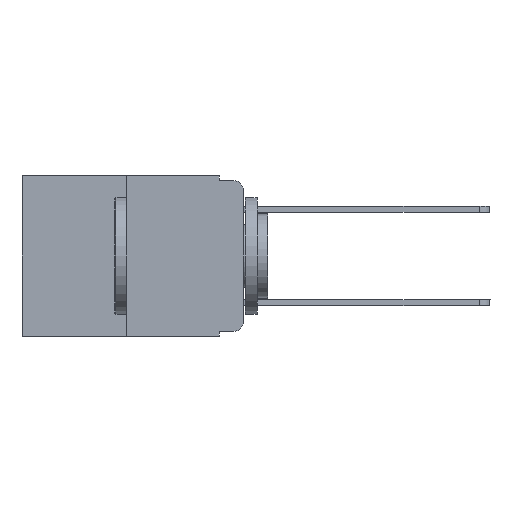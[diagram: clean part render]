
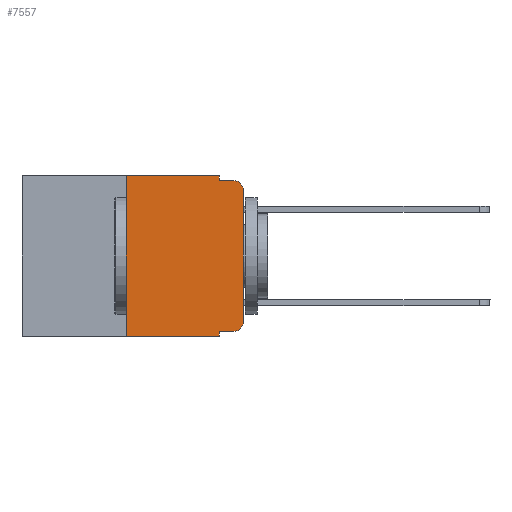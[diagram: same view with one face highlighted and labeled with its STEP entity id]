
A CAD part, left-side view. The second image highlights one B-rep face of the part: STEP entity #7557.
In plain terms, the highlighted planar face has unit normal (-1, 0, 0).
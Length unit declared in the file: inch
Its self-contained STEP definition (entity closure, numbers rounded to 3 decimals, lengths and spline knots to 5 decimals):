
#195 = CARTESIAN_POINT ( 'NONE',  ( 0., 0.051, -0.333 ) ) ;
#1123 = LINE ( 'NONE', #16948, #2028 ) ;
#1170 = CARTESIAN_POINT ( 'NONE',  ( 0., 0., -0.03 ) ) ;
#1408 = ORIENTED_EDGE ( 'NONE', *, *, #11745, .F. ) ;
#1747 = LINE ( 'NONE', #2753, #7333 ) ;
#1785 = LINE ( 'NONE', #195, #9583 ) ;
#2028 = VECTOR ( 'NONE', #9842, 39.37008 ) ;
#2146 = CARTESIAN_POINT ( 'NONE',  ( 0., 0.02, -0.313 ) ) ;
#2162 = VERTEX_POINT ( 'NONE', #2260 ) ;
#2260 = CARTESIAN_POINT ( 'NONE',  ( 0., 0.051, -0.01 ) ) ;
#2746 = EDGE_CURVE ( 'NONE', #6330, #6250, #6515, .T. ) ;
#2752 = EDGE_CURVE ( 'NONE', #5424, #13644, #5398, .T. ) ;
#2753 = CARTESIAN_POINT ( 'NONE',  ( 0., 0.051, -0.01 ) ) ;
#2865 = EDGE_CURVE ( 'NONE', #13417, #8685, #5629, .T. ) ;
#3025 = DIRECTION ( 'NONE',  ( -1., 0., 0. ) ) ;
#3397 = EDGE_CURVE ( 'NONE', #6328, #6330, #1785, .T. ) ;
#3573 = DIRECTION ( 'NONE',  ( -1., 0., 0. ) ) ;
#3875 = DIRECTION ( 'NONE',  ( 0., 0., -1. ) ) ;
#4063 = ORIENTED_EDGE ( 'NONE', *, *, #8047, .F. ) ;
#4667 = EDGE_CURVE ( 'NONE', #6647, #5424, #12189, .T. ) ;
#5398 = LINE ( 'NONE', #17823, #9391 ) ;
#5424 = VERTEX_POINT ( 'NONE', #9596 ) ;
#5507 = ORIENTED_EDGE ( 'NONE', *, *, #3397, .T. ) ;
#5629 = CIRCLE ( 'NONE', #12966, 0.02 ) ;
#5834 = CARTESIAN_POINT ( 'NONE',  ( 0., 0., -0.313 ) ) ;
#5843 = CARTESIAN_POINT ( 'NONE',  ( 0., 0.051, 0. ) ) ;
#6234 = ORIENTED_EDGE ( 'NONE', *, *, #13739, .F. ) ;
#6250 = VERTEX_POINT ( 'NONE', #5834 ) ;
#6328 = VERTEX_POINT ( 'NONE', #15102 ) ;
#6330 = VERTEX_POINT ( 'NONE', #14915 ) ;
#6351 = VECTOR ( 'NONE', #14110, 39.37008 ) ;
#6509 = EDGE_CURVE ( 'NONE', #6250, #13417, #13901, .T. ) ;
#6515 = CIRCLE ( 'NONE', #13325, 0.02 ) ;
#6647 = VERTEX_POINT ( 'NONE', #7744 ) ;
#6911 = CARTESIAN_POINT ( 'NONE',  ( 0., 0.02, -0.01 ) ) ;
#7333 = VECTOR ( 'NONE', #15859, 39.37008 ) ;
#7557 = ADVANCED_FACE ( 'NONE', ( #17306 ), #18148, .F. ) ;
#7744 = CARTESIAN_POINT ( 'NONE',  ( 0., 0.25, -0.343 ) ) ;
#8047 = EDGE_CURVE ( 'NONE', #13644, #2162, #8406, .T. ) ;
#8072 = CARTESIAN_POINT ( 'NONE',  ( 0., 0.25, 0. ) ) ;
#8406 = LINE ( 'NONE', #5843, #15538 ) ;
#8418 = VECTOR ( 'NONE', #10935, 39.37008 ) ;
#8685 = VERTEX_POINT ( 'NONE', #6911 ) ;
#8944 = ORIENTED_EDGE ( 'NONE', *, *, #11287, .T. ) ;
#9391 = VECTOR ( 'NONE', #17770, 39.37008 ) ;
#9583 = VECTOR ( 'NONE', #11407, 39.37008 ) ;
#9596 = CARTESIAN_POINT ( 'NONE',  ( 0., 0.25, 0. ) ) ;
#9811 = VERTEX_POINT ( 'NONE', #10598 ) ;
#9842 = DIRECTION ( 'NONE',  ( 0., 0., -1. ) ) ;
#10598 = CARTESIAN_POINT ( 'NONE',  ( 0., 0.051, -0.343 ) ) ;
#10784 = ORIENTED_EDGE ( 'NONE', *, *, #6509, .T. ) ;
#10935 = DIRECTION ( 'NONE',  ( 0., 0., 1. ) ) ;
#10963 = DIRECTION ( 'NONE',  ( 1., 0., 0. ) ) ;
#11059 = CARTESIAN_POINT ( 'NONE',  ( 0., 0.473, -0.343 ) ) ;
#11287 = EDGE_CURVE ( 'NONE', #6647, #9811, #14077, .T. ) ;
#11328 = ORIENTED_EDGE ( 'NONE', *, *, #2746, .T. ) ;
#11361 = ORIENTED_EDGE ( 'NONE', *, *, #4667, .F. ) ;
#11407 = DIRECTION ( 'NONE',  ( 0., -1., 0. ) ) ;
#11465 = DIRECTION ( 'NONE',  ( 0., 0., -1. ) ) ;
#11745 = EDGE_CURVE ( 'NONE', #6328, #9811, #1123, .T. ) ;
#12189 = LINE ( 'NONE', #8072, #8418 ) ;
#12760 = ORIENTED_EDGE ( 'NONE', *, *, #2752, .F. ) ;
#12966 = AXIS2_PLACEMENT_3D ( 'NONE', #14336, #3025, #14269 ) ;
#13325 = AXIS2_PLACEMENT_3D ( 'NONE', #2146, #3573, #13512 ) ;
#13417 = VERTEX_POINT ( 'NONE', #1170 ) ;
#13512 = DIRECTION ( 'NONE',  ( 0., 0., -1. ) ) ;
#13644 = VERTEX_POINT ( 'NONE', #15751 ) ;
#13739 = EDGE_CURVE ( 'NONE', #2162, #8685, #1747, .T. ) ;
#13901 = LINE ( 'NONE', #16982, #6351 ) ;
#13950 = CARTESIAN_POINT ( 'NONE',  ( 0., 0.473, 0. ) ) ;
#14077 = LINE ( 'NONE', #11059, #16519 ) ;
#14110 = DIRECTION ( 'NONE',  ( 0., 0., 1. ) ) ;
#14269 = DIRECTION ( 'NONE',  ( 0., 0., -1. ) ) ;
#14336 = CARTESIAN_POINT ( 'NONE',  ( 0., 0.02, -0.03 ) ) ;
#14768 = EDGE_LOOP ( 'NONE', ( #10784, #17700, #6234, #4063, #12760, #11361, #8944, #1408, #5507, #11328 ) ) ;
#14915 = CARTESIAN_POINT ( 'NONE',  ( 0., 0.02, -0.333 ) ) ;
#15102 = CARTESIAN_POINT ( 'NONE',  ( 0., 0.051, -0.333 ) ) ;
#15428 = AXIS2_PLACEMENT_3D ( 'NONE', #13950, #10963, #3875 ) ;
#15538 = VECTOR ( 'NONE', #11465, 39.37008 ) ;
#15751 = CARTESIAN_POINT ( 'NONE',  ( 0., 0.051, 0. ) ) ;
#15859 = DIRECTION ( 'NONE',  ( 0., -1., 0. ) ) ;
#16519 = VECTOR ( 'NONE', #18361, 39.37008 ) ;
#16948 = CARTESIAN_POINT ( 'NONE',  ( 0., 0.051, 0. ) ) ;
#16982 = CARTESIAN_POINT ( 'NONE',  ( 0., 0., 0. ) ) ;
#17306 = FACE_OUTER_BOUND ( 'NONE', #14768, .T. ) ;
#17700 = ORIENTED_EDGE ( 'NONE', *, *, #2865, .T. ) ;
#17770 = DIRECTION ( 'NONE',  ( 0., -1., 0. ) ) ;
#17823 = CARTESIAN_POINT ( 'NONE',  ( 0., 0.473, 0. ) ) ;
#18148 = PLANE ( 'NONE',  #15428 ) ;
#18361 = DIRECTION ( 'NONE',  ( 0., -1., 0. ) ) ;
